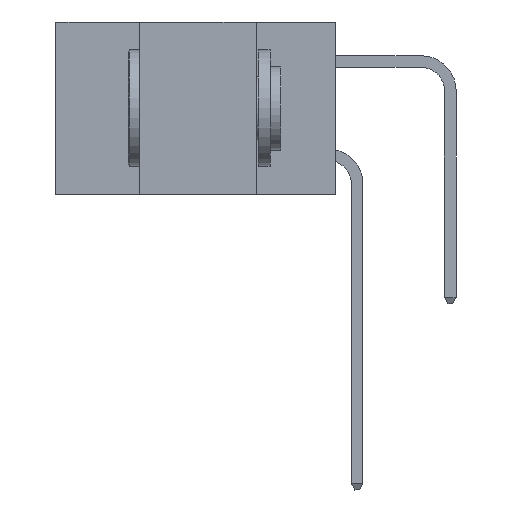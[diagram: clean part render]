
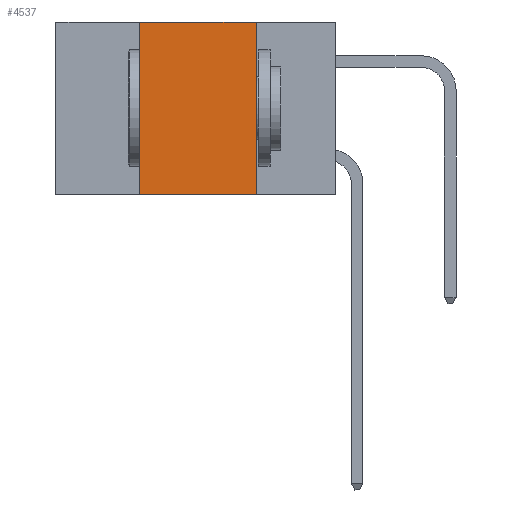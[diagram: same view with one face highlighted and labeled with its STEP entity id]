
A CAD part, left-side view. The second image highlights one B-rep face of the part: STEP entity #4537.
In plain terms, the highlighted planar face has unit normal (-1, 0, 0).
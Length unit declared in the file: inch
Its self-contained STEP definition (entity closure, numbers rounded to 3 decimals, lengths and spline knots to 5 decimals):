
#1095 = PLANE ( 'NONE',  #12266 ) ;
#1718 = LINE ( 'NONE', #10691, #10377 ) ;
#2113 = ORIENTED_EDGE ( 'NONE', *, *, #15350, .T. ) ;
#2308 = VERTEX_POINT ( 'NONE', #21891 ) ;
#2349 = DIRECTION ( 'NONE',  ( 0., 0., -1. ) ) ;
#2723 = ORIENTED_EDGE ( 'NONE', *, *, #5875, .F. ) ;
#3968 = CARTESIAN_POINT ( 'NONE',  ( 0., 0.42, -0.37 ) ) ;
#4537 = ADVANCED_FACE ( 'NONE', ( #18379 ), #1095, .F. ) ;
#4764 = LINE ( 'NONE', #12832, #19389 ) ;
#5787 = CARTESIAN_POINT ( 'NONE',  ( 0., 0.17, 0. ) ) ;
#5875 = EDGE_CURVE ( 'NONE', #23009, #2308, #15824, .T. ) ;
#6806 = EDGE_LOOP ( 'NONE', ( #15315, #20597, #2723, #2113 ) ) ;
#8348 = VECTOR ( 'NONE', #2349, 39.37008 ) ;
#8443 = CARTESIAN_POINT ( 'NONE',  ( 0., 0.6, 0. ) ) ;
#8525 = DIRECTION ( 'NONE',  ( 0., 0., -1. ) ) ;
#8596 = CARTESIAN_POINT ( 'NONE',  ( 0., 0.17, 0. ) ) ;
#8816 = DIRECTION ( 'NONE',  ( 0., -1., 0. ) ) ;
#10377 = VECTOR ( 'NONE', #8816, 39.37008 ) ;
#10691 = CARTESIAN_POINT ( 'NONE',  ( 0., 0.6, 0. ) ) ;
#12144 = EDGE_CURVE ( 'NONE', #2308, #14280, #1718, .T. ) ;
#12266 = AXIS2_PLACEMENT_3D ( 'NONE', #8443, #19527, #8525 ) ;
#12832 = CARTESIAN_POINT ( 'NONE',  ( 0., 0.6, -0.37 ) ) ;
#14280 = VERTEX_POINT ( 'NONE', #5787 ) ;
#14648 = VECTOR ( 'NONE', #16546, 39.37008 ) ;
#15315 = ORIENTED_EDGE ( 'NONE', *, *, #23368, .F. ) ;
#15350 = EDGE_CURVE ( 'NONE', #23009, #21649, #4764, .T. ) ;
#15824 = LINE ( 'NONE', #20083, #14648 ) ;
#16546 = DIRECTION ( 'NONE',  ( 0., 0., 1. ) ) ;
#18379 = FACE_OUTER_BOUND ( 'NONE', #6806, .T. ) ;
#18500 = CARTESIAN_POINT ( 'NONE',  ( 0., 0.17, -0.37 ) ) ;
#19389 = VECTOR ( 'NONE', #23618, 39.37008 ) ;
#19527 = DIRECTION ( 'NONE',  ( 1., 0., 0. ) ) ;
#20083 = CARTESIAN_POINT ( 'NONE',  ( 0., 0.42, 0. ) ) ;
#20597 = ORIENTED_EDGE ( 'NONE', *, *, #12144, .F. ) ;
#21649 = VERTEX_POINT ( 'NONE', #18500 ) ;
#21891 = CARTESIAN_POINT ( 'NONE',  ( 0., 0.42, 0. ) ) ;
#22882 = LINE ( 'NONE', #8596, #8348 ) ;
#23009 = VERTEX_POINT ( 'NONE', #3968 ) ;
#23368 = EDGE_CURVE ( 'NONE', #14280, #21649, #22882, .T. ) ;
#23618 = DIRECTION ( 'NONE',  ( 0., -1., 0. ) ) ;
